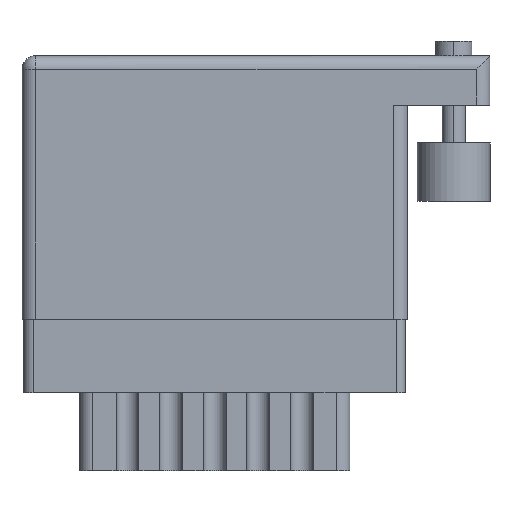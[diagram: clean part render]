
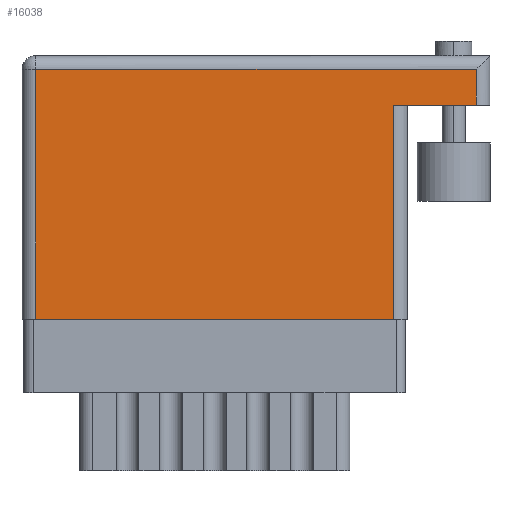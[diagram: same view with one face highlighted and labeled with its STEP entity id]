
A CAD part, front view. The second image highlights one B-rep face of the part: STEP entity #16038.
In plain terms, the highlighted face is planar.
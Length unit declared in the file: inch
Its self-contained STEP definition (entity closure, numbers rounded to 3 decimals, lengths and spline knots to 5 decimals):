
#373 = ORIENTED_EDGE ( 'NONE', *, *, #15472, .T. ) ;
#837 = ORIENTED_EDGE ( 'NONE', *, *, #16490, .T. ) ;
#1375 = VECTOR ( 'NONE', #13142, 39.37008 ) ;
#1613 = LINE ( 'NONE', #7620, #19531 ) ;
#2453 = LINE ( 'NONE', #5860, #13680 ) ;
#2790 = LINE ( 'NONE', #8057, #3908 ) ;
#2811 = CARTESIAN_POINT ( 'NONE',  ( 0.047, 0.859, 0. ) ) ;
#3892 = LINE ( 'NONE', #13775, #7690 ) ;
#3908 = VECTOR ( 'NONE', #23656, 39.37008 ) ;
#4208 = LINE ( 'NONE', #6290, #4579 ) ;
#4273 = VERTEX_POINT ( 'NONE', #22699 ) ;
#4513 = EDGE_CURVE ( 'NONE', #6714, #6294, #4208, .T. ) ;
#4579 = VECTOR ( 'NONE', #8624, 39.37008 ) ;
#5664 = DIRECTION ( 'NONE',  ( -1., 0., 0. ) ) ;
#5860 = CARTESIAN_POINT ( 'NONE',  ( 0.047, 0., 0. ) ) ;
#6126 = PLANE ( 'NONE',  #9745 ) ;
#6290 = CARTESIAN_POINT ( 'NONE',  ( 1.562, 0.906, 0. ) ) ;
#6294 = VERTEX_POINT ( 'NONE', #18716 ) ;
#6714 = VERTEX_POINT ( 'NONE', #23484 ) ;
#6724 = EDGE_CURVE ( 'NONE', #6294, #12780, #1613, .T. ) ;
#6774 = CARTESIAN_POINT ( 'NONE',  ( 0., 0., 0. ) ) ;
#6854 = ORIENTED_EDGE ( 'NONE', *, *, #4513, .T. ) ;
#7175 = EDGE_CURVE ( 'NONE', #12780, #4273, #2453, .T. ) ;
#7620 = CARTESIAN_POINT ( 'NONE',  ( 0., 0.859, 0. ) ) ;
#7690 = VECTOR ( 'NONE', #21208, 39.37008 ) ;
#8057 = CARTESIAN_POINT ( 'NONE',  ( 1.278, 0.736, 0. ) ) ;
#8624 = DIRECTION ( 'NONE',  ( 0., 1., 0. ) ) ;
#8976 = CARTESIAN_POINT ( 'NONE',  ( 1.278, 0., 0. ) ) ;
#9745 = AXIS2_PLACEMENT_3D ( 'NONE', #14057, #21996, #12246 ) ;
#10795 = LINE ( 'NONE', #6774, #1375 ) ;
#10860 = CARTESIAN_POINT ( 'NONE',  ( 1.278, 0.736, 0. ) ) ;
#12246 = DIRECTION ( 'NONE',  ( -1., 0., 0. ) ) ;
#12496 = ORIENTED_EDGE ( 'NONE', *, *, #6724, .T. ) ;
#12780 = VERTEX_POINT ( 'NONE', #2811 ) ;
#13142 = DIRECTION ( 'NONE',  ( 1., 0., 0. ) ) ;
#13680 = VECTOR ( 'NONE', #13789, 39.37008 ) ;
#13775 = CARTESIAN_POINT ( 'NONE',  ( 1.609, 0.736, 0. ) ) ;
#13789 = DIRECTION ( 'NONE',  ( 0., -1., 0. ) ) ;
#14057 = CARTESIAN_POINT ( 'NONE',  ( 0., 0.906, 0. ) ) ;
#14544 = VERTEX_POINT ( 'NONE', #10860 ) ;
#15472 = EDGE_CURVE ( 'NONE', #4273, #16139, #10795, .T. ) ;
#16038 = ADVANCED_FACE ( 'NONE', ( #23954 ), #6126, .F. ) ;
#16139 = VERTEX_POINT ( 'NONE', #8976 ) ;
#16490 = EDGE_CURVE ( 'NONE', #16139, #14544, #2790, .T. ) ;
#17612 = EDGE_CURVE ( 'NONE', #6714, #14544, #3892, .T. ) ;
#18716 = CARTESIAN_POINT ( 'NONE',  ( 1.562, 0.859, 0. ) ) ;
#18943 = ORIENTED_EDGE ( 'NONE', *, *, #7175, .T. ) ;
#19323 = EDGE_LOOP ( 'NONE', ( #373, #837, #22602, #6854, #12496, #18943 ) ) ;
#19531 = VECTOR ( 'NONE', #5664, 39.37008 ) ;
#21208 = DIRECTION ( 'NONE',  ( -1., 0., 0. ) ) ;
#21996 = DIRECTION ( 'NONE',  ( 0., 0., -1. ) ) ;
#22602 = ORIENTED_EDGE ( 'NONE', *, *, #17612, .F. ) ;
#22699 = CARTESIAN_POINT ( 'NONE',  ( 0.047, 0., 0. ) ) ;
#23484 = CARTESIAN_POINT ( 'NONE',  ( 1.562, 0.736, 0. ) ) ;
#23656 = DIRECTION ( 'NONE',  ( 0., 1., 0. ) ) ;
#23954 = FACE_OUTER_BOUND ( 'NONE', #19323, .T. ) ;
